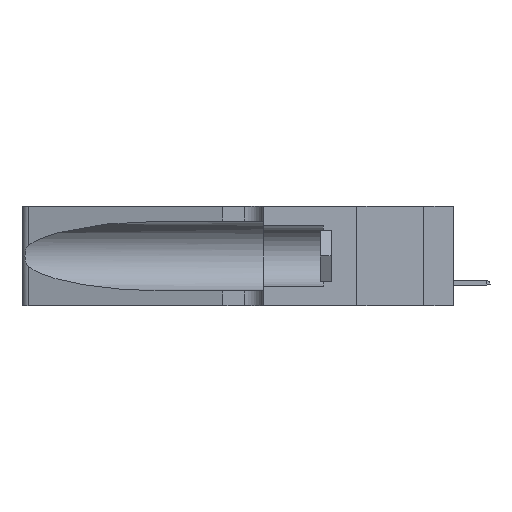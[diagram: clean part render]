
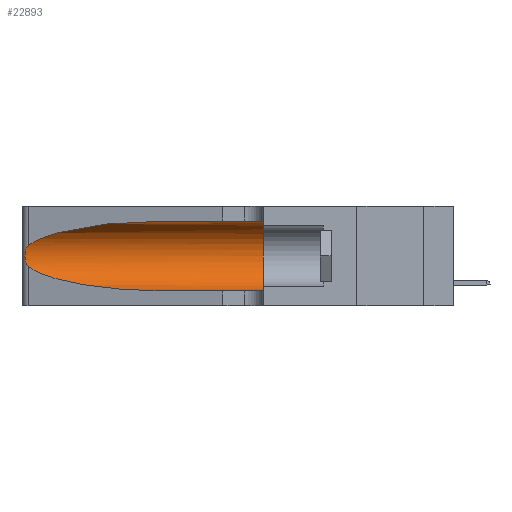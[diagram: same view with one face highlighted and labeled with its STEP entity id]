
A CAD part, left-side view. The second image highlights one B-rep face of the part: STEP entity #22893.
In plain terms, the highlighted cylindrical face has radius 3.308 mm (diameter 6.617 mm), a partial arc.
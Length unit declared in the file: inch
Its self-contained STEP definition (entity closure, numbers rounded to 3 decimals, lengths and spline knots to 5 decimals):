
#13 =( BOUNDED_CURVE ( )  B_SPLINE_CURVE ( 3, ( #42247, #7337, #4385, #31713 ),
 .UNSPECIFIED., .F., .T. ) 
 B_SPLINE_CURVE_WITH_KNOTS ( ( 4, 4 ),
 ( 3.44316, 4.71239 ),
 .UNSPECIFIED. ) 
 CURVE ( )  GEOMETRIC_REPRESENTATION_ITEM ( )  RATIONAL_B_SPLINE_CURVE ( ( 1., 0.87, 0.87, 1. ) ) 
 REPRESENTATION_ITEM ( '' )  );
#966 = DIRECTION ( 'NONE',  ( 0., 0., 1. ) ) ;
#1369 = CARTESIAN_POINT ( 'NONE',  ( 0.1305, 0.72297, 0.31525 ) ) ;
#1699 = EDGE_CURVE ( 'NONE', #7827, #18063, #25210, .T. ) ;
#2578 = EDGE_CURVE ( 'NONE', #7529, #19122, #8724, .T. ) ;
#3282 = CARTESIAN_POINT ( 'NONE',  ( 0.1305, 0.72297, 0.05475 ) ) ;
#3890 = CARTESIAN_POINT ( 'NONE',  ( 0.25789, 1.23486, 0.15765 ) ) ;
#4132 = FACE_OUTER_BOUND ( 'NONE', #8520, .T. ) ;
#4385 = CARTESIAN_POINT ( 'NONE',  ( 0.18966, 0.96281, 0.05475 ) ) ;
#4841 = CARTESIAN_POINT ( 'NONE',  ( 0.18966, 0.96281, 0.31525 ) ) ;
#4963 = EDGE_CURVE ( 'NONE', #27131, #22163, #31139, .T. ) ;
#5758 = CARTESIAN_POINT ( 'NONE',  ( 0.1305, 1.61858, 0.31525 ) ) ;
#7337 = CARTESIAN_POINT ( 'NONE',  ( 0.2373, 1.15595, 0.08982 ) ) ;
#7529 = VERTEX_POINT ( 'NONE', #1369 ) ;
#7827 = VERTEX_POINT ( 'NONE', #42375 ) ;
#7880 = ORIENTED_EDGE ( 'NONE', *, *, #43429, .F. ) ;
#8520 = EDGE_LOOP ( 'NONE', ( #38517, #24984, #15380, #15901, #7880, #31780 ) ) ;
#8724 = LINE ( 'NONE', #5758, #44210 ) ;
#10463 = CARTESIAN_POINT ( 'NONE',  ( 0.25787, 1.23484, 0.2124 ) ) ;
#11142 = CARTESIAN_POINT ( 'NONE',  ( 0.25856, 1.23593, 0.16098 ) ) ;
#11648 = CARTESIAN_POINT ( 'NONE',  ( 0.2373, 1.15595, 0.28018 ) ) ;
#14326 = CARTESIAN_POINT ( 'NONE',  ( 0.26075, 1.23896, 0.19203 ) ) ;
#15213 = EDGE_CURVE ( 'NONE', #18063, #27131, #13, .T. ) ;
#15380 = ORIENTED_EDGE ( 'NONE', *, *, #15213, .T. ) ;
#15901 = ORIENTED_EDGE ( 'NONE', *, *, #4963, .T. ) ;
#16221 = DIRECTION ( 'NONE',  ( 0., -1., 0. ) ) ;
#16808 = CARTESIAN_POINT ( 'NONE',  ( 0.25487, 1.22718, 0.14631 ) ) ;
#17109 = CYLINDRICAL_SURFACE ( 'NONE', #22324, 0.13025 ) ;
#18063 = VERTEX_POINT ( 'NONE', #16808 ) ;
#18486 = CARTESIAN_POINT ( 'NONE',  ( 0.1305, 0.72297, 0.31525 ) ) ;
#18494 = CARTESIAN_POINT ( 'NONE',  ( 0.1305, 0.35, 0.185 ) ) ;
#18676 =( BOUNDED_CURVE ( )  B_SPLINE_CURVE ( 3, ( #18486, #4841, #11648, #38801 ),
 .UNSPECIFIED., .F., .T. ) 
 B_SPLINE_CURVE_WITH_KNOTS ( ( 4, 4 ),
 ( 1.5708, 2.84003 ),
 .UNSPECIFIED. ) 
 CURVE ( )  GEOMETRIC_REPRESENTATION_ITEM ( )  RATIONAL_B_SPLINE_CURVE ( ( 1., 0.87, 0.87, 1. ) ) 
 REPRESENTATION_ITEM ( '' )  );
#19122 = VERTEX_POINT ( 'NONE', #21159 ) ;
#21159 = CARTESIAN_POINT ( 'NONE',  ( 0.1305, 0.35, 0.31525 ) ) ;
#22084 = VECTOR ( 'NONE', #41202, 39.37008 ) ;
#22163 = VERTEX_POINT ( 'NONE', #28397 ) ;
#22324 = AXIS2_PLACEMENT_3D ( 'NONE', #35137, #41999, #37886 ) ;
#22893 = ADVANCED_FACE ( 'NONE', ( #4132 ), #17109, .F. ) ;
#24374 = CARTESIAN_POINT ( 'NONE',  ( 0.25639, 1.23186, 0.15144 ) ) ;
#24849 = CARTESIAN_POINT ( 'NONE',  ( 0.25487, 1.22718, 0.14631 ) ) ;
#24984 = ORIENTED_EDGE ( 'NONE', *, *, #1699, .T. ) ;
#25210 = B_SPLINE_CURVE_WITH_KNOTS ( 'NONE', 3,
 ( #31911, #35577, #27809, #10463, #35334, #28494, #14326, #35119, #31677, #11142, #3890, #24374, #28268, #24849 ),
 .UNSPECIFIED., .F., .F.,
 ( 4, 2, 2, 2, 2, 2, 4 ),
 ( 0., 0.00027, 0.00053, 0.00107, 0.0016, 0.00187, 0.00214 ),
 .UNSPECIFIED. ) ;
#27131 = VERTEX_POINT ( 'NONE', #3282 ) ;
#27809 = CARTESIAN_POINT ( 'NONE',  ( 0.25639, 1.23184, 0.21858 ) ) ;
#28268 = CARTESIAN_POINT ( 'NONE',  ( 0.25555, 1.22993, 0.14849 ) ) ;
#28397 = CARTESIAN_POINT ( 'NONE',  ( 0.1305, 0.35, 0.05475 ) ) ;
#28494 = CARTESIAN_POINT ( 'NONE',  ( 0.26018, 1.23835, 0.19895 ) ) ;
#29024 = EDGE_CURVE ( 'NONE', #7529, #7827, #18676, .T. ) ;
#29321 = CIRCLE ( 'NONE', #35127, 0.13025 ) ;
#31139 = LINE ( 'NONE', #34126, #22084 ) ;
#31677 = CARTESIAN_POINT ( 'NONE',  ( 0.26017, 1.23833, 0.17102 ) ) ;
#31713 = CARTESIAN_POINT ( 'NONE',  ( 0.1305, 0.72297, 0.05475 ) ) ;
#31780 = ORIENTED_EDGE ( 'NONE', *, *, #2578, .F. ) ;
#31911 = CARTESIAN_POINT ( 'NONE',  ( 0.25487, 1.22718, 0.22369 ) ) ;
#34126 = CARTESIAN_POINT ( 'NONE',  ( 0.1305, 1.61858, 0.05475 ) ) ;
#35119 = CARTESIAN_POINT ( 'NONE',  ( 0.26075, 1.23896, 0.178 ) ) ;
#35127 = AXIS2_PLACEMENT_3D ( 'NONE', #18494, #35624, #966 ) ;
#35137 = CARTESIAN_POINT ( 'NONE',  ( 0.1305, 1.61858, 0.185 ) ) ;
#35334 = CARTESIAN_POINT ( 'NONE',  ( 0.25854, 1.2359, 0.20912 ) ) ;
#35577 = CARTESIAN_POINT ( 'NONE',  ( 0.25555, 1.22994, 0.2215 ) ) ;
#35624 = DIRECTION ( 'NONE',  ( 0., 1., 0. ) ) ;
#37886 = DIRECTION ( 'NONE',  ( 0., 0., -1. ) ) ;
#38517 = ORIENTED_EDGE ( 'NONE', *, *, #29024, .T. ) ;
#38801 = CARTESIAN_POINT ( 'NONE',  ( 0.25487, 1.22718, 0.22369 ) ) ;
#41202 = DIRECTION ( 'NONE',  ( 0., -1., 0. ) ) ;
#41999 = DIRECTION ( 'NONE',  ( 0., -1., 0. ) ) ;
#42247 = CARTESIAN_POINT ( 'NONE',  ( 0.25487, 1.22718, 0.14631 ) ) ;
#42375 = CARTESIAN_POINT ( 'NONE',  ( 0.25487, 1.22718, 0.22369 ) ) ;
#43429 = EDGE_CURVE ( 'NONE', #19122, #22163, #29321, .T. ) ;
#44210 = VECTOR ( 'NONE', #16221, 39.37008 ) ;
